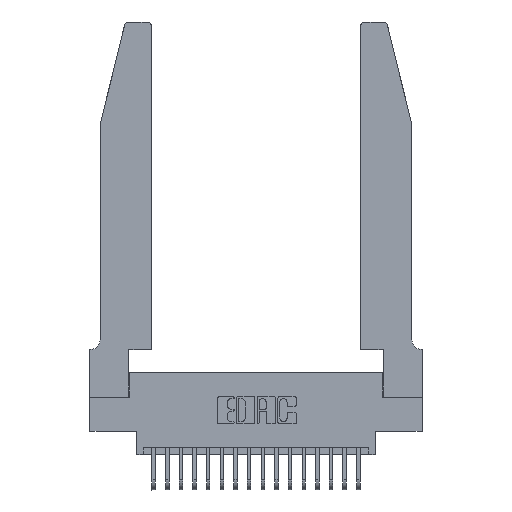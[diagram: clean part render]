
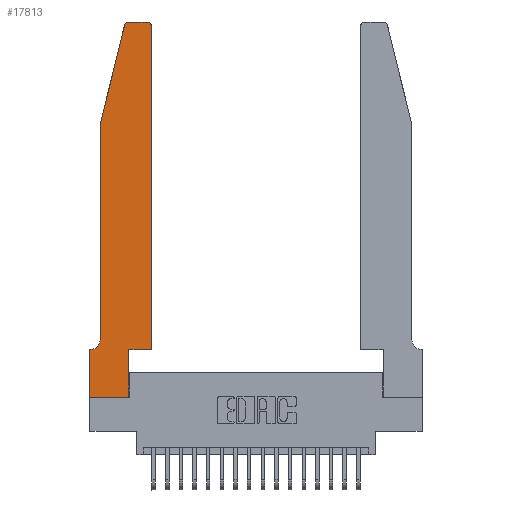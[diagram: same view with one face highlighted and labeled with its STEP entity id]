
A CAD part, top view. The second image highlights one B-rep face of the part: STEP entity #17813.
In plain terms, the highlighted planar face has unit normal (0, 0, 1).
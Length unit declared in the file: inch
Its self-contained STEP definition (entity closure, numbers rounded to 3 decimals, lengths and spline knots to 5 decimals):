
#14 = AXIS2_PLACEMENT_3D ( 'NONE', #17516, #8069, #19067 ) ;
#76 = LINE ( 'NONE', #5684, #15520 ) ;
#279 = VERTEX_POINT ( 'NONE', #16700 ) ;
#365 = ORIENTED_EDGE ( 'NONE', *, *, #20444, .T. ) ;
#449 = CARTESIAN_POINT ( 'NONE',  ( 0.0755, 2., 0.37 ) ) ;
#697 = CARTESIAN_POINT ( 'NONE',  ( 0., 0.35, 0.37 ) ) ;
#701 = LINE ( 'NONE', #13726, #16615 ) ;
#769 = EDGE_CURVE ( 'NONE', #10407, #7466, #20479, .T. ) ;
#969 = DIRECTION ( 'NONE',  ( 0., 0., 1. ) ) ;
#1301 = CARTESIAN_POINT ( 'NONE',  ( 0.0755, 0.35, 0.37 ) ) ;
#1533 = EDGE_CURVE ( 'NONE', #16992, #15992, #19242, .T. ) ;
#1579 = CARTESIAN_POINT ( 'NONE',  ( 0.0755, 2., 0.37 ) ) ;
#1758 = CARTESIAN_POINT ( 'NONE',  ( 0.0755, 2., 0.37 ) ) ;
#1811 = VERTEX_POINT ( 'NONE', #4037 ) ;
#1865 = EDGE_CURVE ( 'NONE', #1811, #5284, #11122, .T. ) ;
#1923 = CARTESIAN_POINT ( 'NONE',  ( 0.4505, 0.35, 0.37 ) ) ;
#2319 = DIRECTION ( 'NONE',  ( 0., 0., 1. ) ) ;
#2417 = VECTOR ( 'NONE', #14484, 39.37008 ) ;
#2464 = DIRECTION ( 'NONE',  ( 0., -1., 0. ) ) ;
#2977 = DIRECTION ( 'NONE',  ( 1., 0., 0. ) ) ;
#3512 = VECTOR ( 'NONE', #18423, 39.37008 ) ;
#3680 = DIRECTION ( 'NONE',  ( -0.239, -0.971, 0. ) ) ;
#3807 = AXIS2_PLACEMENT_3D ( 'NONE', #10520, #969, #12125 ) ;
#4037 = CARTESIAN_POINT ( 'NONE',  ( 0.4505, 2.72, 0.37 ) ) ;
#4946 = LINE ( 'NONE', #1923, #16591 ) ;
#5068 = VERTEX_POINT ( 'NONE', #16727 ) ;
#5284 = VERTEX_POINT ( 'NONE', #14390 ) ;
#5345 = EDGE_CURVE ( 'NONE', #5068, #20500, #12738, .T. ) ;
#5684 = CARTESIAN_POINT ( 'NONE',  ( 0., 0., 0.37 ) ) ;
#5744 = CARTESIAN_POINT ( 'NONE',  ( 0.4505, 0.35, 0.37 ) ) ;
#6114 = EDGE_CURVE ( 'NONE', #7466, #12278, #11989, .T. ) ;
#6466 = EDGE_CURVE ( 'NONE', #279, #1811, #4946, .T. ) ;
#6851 = LINE ( 'NONE', #1301, #14751 ) ;
#6996 = VECTOR ( 'NONE', #3680, 39.37008 ) ;
#7374 = VERTEX_POINT ( 'NONE', #15756 ) ;
#7466 = VERTEX_POINT ( 'NONE', #13973 ) ;
#7668 = LINE ( 'NONE', #5744, #15061 ) ;
#8069 = DIRECTION ( 'NONE',  ( 0., 0., -1. ) ) ;
#8255 = CARTESIAN_POINT ( 'NONE',  ( 0.284, 2.72, 0.37 ) ) ;
#8944 = DIRECTION ( 'NONE',  ( 1., 0., 0. ) ) ;
#9043 = DIRECTION ( 'NONE',  ( -1., 0., 0. ) ) ;
#9249 = CARTESIAN_POINT ( 'NONE',  ( 0.0755, 0.42, 0.37 ) ) ;
#9260 = DIRECTION ( 'NONE',  ( -1., 0., 0. ) ) ;
#9387 = CARTESIAN_POINT ( 'NONE',  ( 0.25487, 2.72718, 0.37 ) ) ;
#9823 = DIRECTION ( 'NONE',  ( 1., 0., 0. ) ) ;
#10407 = VERTEX_POINT ( 'NONE', #14888 ) ;
#10520 = CARTESIAN_POINT ( 'NONE',  ( 0.4205, 2.72, 0.37 ) ) ;
#10676 = ORIENTED_EDGE ( 'NONE', *, *, #6466, .T. ) ;
#10932 = CARTESIAN_POINT ( 'NONE',  ( 0., 0., 0.37 ) ) ;
#11030 = CARTESIAN_POINT ( 'NONE',  ( 0.0055, 0.35, 0.37 ) ) ;
#11122 = CIRCLE ( 'NONE', #3807, 0.03 ) ;
#11200 = AXIS2_PLACEMENT_3D ( 'NONE', #8255, #19240, #9823 ) ;
#11226 = ORIENTED_EDGE ( 'NONE', *, *, #1865, .T. ) ;
#11241 = ORIENTED_EDGE ( 'NONE', *, *, #1533, .T. ) ;
#11615 = FACE_OUTER_BOUND ( 'NONE', #16520, .T. ) ;
#11665 = CIRCLE ( 'NONE', #14, 0.07 ) ;
#11713 = ORIENTED_EDGE ( 'NONE', *, *, #13331, .T. ) ;
#11778 = ORIENTED_EDGE ( 'NONE', *, *, #14240, .T. ) ;
#11989 = LINE ( 'NONE', #16783, #3512 ) ;
#12125 = DIRECTION ( 'NONE',  ( 1., 0., 0. ) ) ;
#12164 = VECTOR ( 'NONE', #2977, 39.37008 ) ;
#12278 = VERTEX_POINT ( 'NONE', #16432 ) ;
#12738 = CIRCLE ( 'NONE', #11200, 0.03 ) ;
#12805 = ORIENTED_EDGE ( 'NONE', *, *, #769, .T. ) ;
#13027 = DIRECTION ( 'NONE',  ( 0., 1., 0. ) ) ;
#13331 = EDGE_CURVE ( 'NONE', #20500, #16992, #19532, .T. ) ;
#13361 = ORIENTED_EDGE ( 'NONE', *, *, #13473, .T. ) ;
#13418 = DIRECTION ( 'NONE',  ( 1., 0., 0. ) ) ;
#13473 = EDGE_CURVE ( 'NONE', #5284, #5068, #701, .T. ) ;
#13726 = CARTESIAN_POINT ( 'NONE',  ( 0.2605, 2.75, 0.37 ) ) ;
#13973 = CARTESIAN_POINT ( 'NONE',  ( 0.2865, 0., 0.37 ) ) ;
#14240 = EDGE_CURVE ( 'NONE', #15992, #19330, #11665, .T. ) ;
#14390 = CARTESIAN_POINT ( 'NONE',  ( 0.4205, 2.75, 0.37 ) ) ;
#14484 = DIRECTION ( 'NONE',  ( 0., -1., 0. ) ) ;
#14751 = VECTOR ( 'NONE', #9260, 39.37008 ) ;
#14877 = AXIS2_PLACEMENT_3D ( 'NONE', #697, #2319, #13418 ) ;
#14888 = CARTESIAN_POINT ( 'NONE',  ( 0., 0., 0.37 ) ) ;
#14945 = ORIENTED_EDGE ( 'NONE', *, *, #6114, .T. ) ;
#15061 = VECTOR ( 'NONE', #8944, 39.37008 ) ;
#15460 = EDGE_CURVE ( 'NONE', #12278, #279, #7668, .T. ) ;
#15471 = ORIENTED_EDGE ( 'NONE', *, *, #5345, .T. ) ;
#15520 = VECTOR ( 'NONE', #2464, 39.37008 ) ;
#15756 = CARTESIAN_POINT ( 'NONE',  ( 0., 0.35, 0.37 ) ) ;
#15992 = VERTEX_POINT ( 'NONE', #9249 ) ;
#16432 = CARTESIAN_POINT ( 'NONE',  ( 0.2865, 0.35, 0.37 ) ) ;
#16520 = EDGE_LOOP ( 'NONE', ( #13361, #15471, #11713, #11241, #11778, #365, #18908, #12805, #14945, #16706, #10676, #11226 ) ) ;
#16591 = VECTOR ( 'NONE', #13027, 39.37008 ) ;
#16615 = VECTOR ( 'NONE', #9043, 39.37008 ) ;
#16700 = CARTESIAN_POINT ( 'NONE',  ( 0.4505, 0.35, 0.37 ) ) ;
#16706 = ORIENTED_EDGE ( 'NONE', *, *, #15460, .T. ) ;
#16727 = CARTESIAN_POINT ( 'NONE',  ( 0.284, 2.75, 0.37 ) ) ;
#16783 = CARTESIAN_POINT ( 'NONE',  ( 0.2865, 0.35, 0.37 ) ) ;
#16992 = VERTEX_POINT ( 'NONE', #1579 ) ;
#17516 = CARTESIAN_POINT ( 'NONE',  ( 0.0055, 0.42, 0.37 ) ) ;
#17813 = ADVANCED_FACE ( 'NONE', ( #11615 ), #18134, .T. ) ;
#18134 = PLANE ( 'NONE',  #14877 ) ;
#18423 = DIRECTION ( 'NONE',  ( 0., 1., 0. ) ) ;
#18908 = ORIENTED_EDGE ( 'NONE', *, *, #19691, .T. ) ;
#19067 = DIRECTION ( 'NONE',  ( -1., 0., 0. ) ) ;
#19240 = DIRECTION ( 'NONE',  ( 0., 0., 1. ) ) ;
#19242 = LINE ( 'NONE', #1758, #2417 ) ;
#19330 = VERTEX_POINT ( 'NONE', #11030 ) ;
#19532 = LINE ( 'NONE', #449, #6996 ) ;
#19691 = EDGE_CURVE ( 'NONE', #7374, #10407, #76, .T. ) ;
#20444 = EDGE_CURVE ( 'NONE', #19330, #7374, #6851, .T. ) ;
#20479 = LINE ( 'NONE', #10932, #12164 ) ;
#20500 = VERTEX_POINT ( 'NONE', #9387 ) ;
